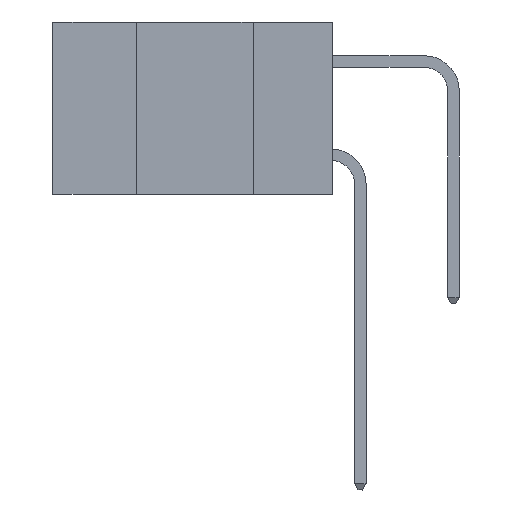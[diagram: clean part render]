
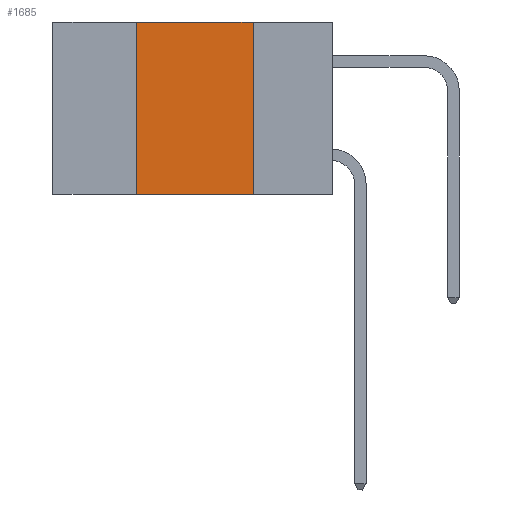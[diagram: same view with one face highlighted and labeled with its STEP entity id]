
A CAD part, left-side view. The second image highlights one B-rep face of the part: STEP entity #1685.
In plain terms, the highlighted planar face has unit normal (-1, 0, 0).
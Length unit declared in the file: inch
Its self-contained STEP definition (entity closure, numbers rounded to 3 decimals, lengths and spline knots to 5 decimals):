
#226 = LINE ( 'NONE', #16936, #18216 ) ;
#496 = DIRECTION ( 'NONE',  ( 0., 0., -1. ) ) ;
#1685 = ADVANCED_FACE ( 'NONE', ( #8468 ), #26824, .F. ) ;
#3484 = EDGE_CURVE ( 'NONE', #4811, #8575, #27205, .T. ) ;
#4811 = VERTEX_POINT ( 'NONE', #29043 ) ;
#5224 = CARTESIAN_POINT ( 'NONE',  ( 0., 0.17, 0. ) ) ;
#6393 = CARTESIAN_POINT ( 'NONE',  ( 0., 0.6, 0. ) ) ;
#6592 = LINE ( 'NONE', #5224, #25139 ) ;
#7128 = DIRECTION ( 'NONE',  ( 0., -1., 0. ) ) ;
#8468 = FACE_OUTER_BOUND ( 'NONE', #20695, .T. ) ;
#8575 = VERTEX_POINT ( 'NONE', #29129 ) ;
#12224 = ORIENTED_EDGE ( 'NONE', *, *, #14083, .F. ) ;
#13652 = ORIENTED_EDGE ( 'NONE', *, *, #21333, .F. ) ;
#14083 = EDGE_CURVE ( 'NONE', #4811, #18980, #226, .T. ) ;
#14968 = ORIENTED_EDGE ( 'NONE', *, *, #3484, .T. ) ;
#16936 = CARTESIAN_POINT ( 'NONE',  ( 0., 0.42, 0. ) ) ;
#16992 = VECTOR ( 'NONE', #22728, 39.37008 ) ;
#18216 = VECTOR ( 'NONE', #19263, 39.37008 ) ;
#18980 = VERTEX_POINT ( 'NONE', #22751 ) ;
#19263 = DIRECTION ( 'NONE',  ( 0., 0., 1. ) ) ;
#19302 = ORIENTED_EDGE ( 'NONE', *, *, #19549, .F. ) ;
#19549 = EDGE_CURVE ( 'NONE', #18980, #21007, #28383, .T. ) ;
#20492 = DIRECTION ( 'NONE',  ( 0., 0., -1. ) ) ;
#20695 = EDGE_LOOP ( 'NONE', ( #13652, #19302, #12224, #14968 ) ) ;
#21007 = VERTEX_POINT ( 'NONE', #27572 ) ;
#21333 = EDGE_CURVE ( 'NONE', #21007, #8575, #6592, .T. ) ;
#22728 = DIRECTION ( 'NONE',  ( 0., -1., 0. ) ) ;
#22751 = CARTESIAN_POINT ( 'NONE',  ( 0., 0.42, 0. ) ) ;
#23453 = CARTESIAN_POINT ( 'NONE',  ( 0., 0.6, -0.37 ) ) ;
#24307 = DIRECTION ( 'NONE',  ( 1., 0., 0. ) ) ;
#24888 = CARTESIAN_POINT ( 'NONE',  ( 0., 0.6, 0. ) ) ;
#25139 = VECTOR ( 'NONE', #496, 39.37008 ) ;
#26518 = VECTOR ( 'NONE', #7128, 39.37008 ) ;
#26824 = PLANE ( 'NONE',  #28355 ) ;
#27205 = LINE ( 'NONE', #23453, #26518 ) ;
#27572 = CARTESIAN_POINT ( 'NONE',  ( 0., 0.17, 0. ) ) ;
#28355 = AXIS2_PLACEMENT_3D ( 'NONE', #24888, #24307, #20492 ) ;
#28383 = LINE ( 'NONE', #6393, #16992 ) ;
#29043 = CARTESIAN_POINT ( 'NONE',  ( 0., 0.42, -0.37 ) ) ;
#29129 = CARTESIAN_POINT ( 'NONE',  ( 0., 0.17, -0.37 ) ) ;
